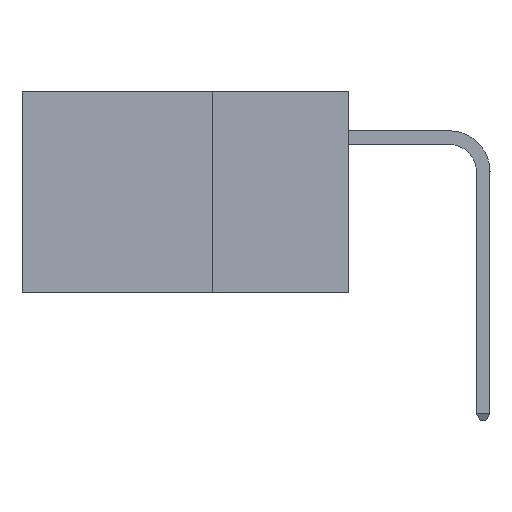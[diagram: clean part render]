
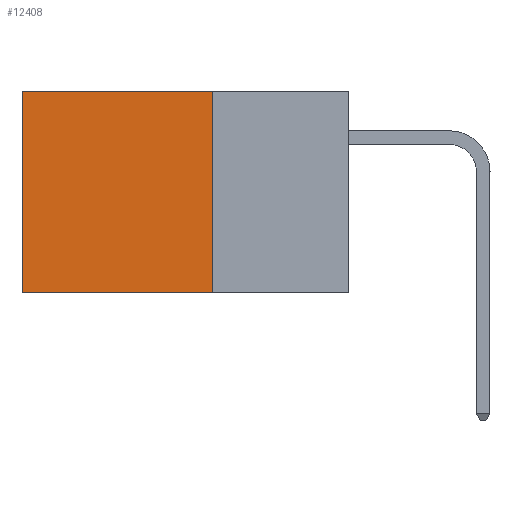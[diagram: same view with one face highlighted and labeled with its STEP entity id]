
A CAD part, left-side view. The second image highlights one B-rep face of the part: STEP entity #12408.
In plain terms, the highlighted planar face has unit normal (-1, 0, 0).
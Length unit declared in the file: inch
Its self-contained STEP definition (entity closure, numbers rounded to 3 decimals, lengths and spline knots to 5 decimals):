
#170 = ORIENTED_EDGE ( 'NONE', *, *, #18555, .F. ) ;
#573 = PLANE ( 'NONE',  #17399 ) ;
#2925 = VECTOR ( 'NONE', #14202, 39.37008 ) ;
#3123 = CARTESIAN_POINT ( 'NONE',  ( 0.2875, 0.25, 0. ) ) ;
#3824 = VECTOR ( 'NONE', #7784, 39.37008 ) ;
#4031 = EDGE_CURVE ( 'NONE', #7311, #18644, #6865, .T. ) ;
#4388 = LINE ( 'NONE', #3123, #8289 ) ;
#5728 = EDGE_CURVE ( 'NONE', #7311, #11360, #4388, .T. ) ;
#6865 = LINE ( 'NONE', #9931, #2925 ) ;
#7175 = CARTESIAN_POINT ( 'NONE',  ( 0.2875, 0.25, -0.37 ) ) ;
#7311 = VERTEX_POINT ( 'NONE', #15298 ) ;
#7784 = DIRECTION ( 'NONE',  ( 0., 1., 0. ) ) ;
#8061 = DIRECTION ( 'NONE',  ( 1., 0., 0. ) ) ;
#8214 = ORIENTED_EDGE ( 'NONE', *, *, #5728, .F. ) ;
#8289 = VECTOR ( 'NONE', #11822, 39.37008 ) ;
#9931 = CARTESIAN_POINT ( 'NONE',  ( 0.2875, 0.25, 0. ) ) ;
#10658 = LINE ( 'NONE', #16256, #3824 ) ;
#11360 = VERTEX_POINT ( 'NONE', #7175 ) ;
#11436 = CARTESIAN_POINT ( 'NONE',  ( 0.2875, 0.6, 0. ) ) ;
#11729 = FACE_OUTER_BOUND ( 'NONE', #13783, .T. ) ;
#11822 = DIRECTION ( 'NONE',  ( 0., 0., -1. ) ) ;
#12408 = ADVANCED_FACE ( 'NONE', ( #11729 ), #573, .F. ) ;
#12698 = ORIENTED_EDGE ( 'NONE', *, *, #18350, .T. ) ;
#12772 = CARTESIAN_POINT ( 'NONE',  ( 0.2875, 0.6, -0.37 ) ) ;
#13235 = VERTEX_POINT ( 'NONE', #12772 ) ;
#13783 = EDGE_LOOP ( 'NONE', ( #12698, #170, #8214, #15871 ) ) ;
#14202 = DIRECTION ( 'NONE',  ( 0., 1., 0. ) ) ;
#14650 = LINE ( 'NONE', #11436, #17878 ) ;
#15109 = CARTESIAN_POINT ( 'NONE',  ( 0.2875, 0.6, 0. ) ) ;
#15298 = CARTESIAN_POINT ( 'NONE',  ( 0.2875, 0.25, 0. ) ) ;
#15871 = ORIENTED_EDGE ( 'NONE', *, *, #4031, .T. ) ;
#16256 = CARTESIAN_POINT ( 'NONE',  ( 0.2875, 0.25, -0.37 ) ) ;
#16524 = CARTESIAN_POINT ( 'NONE',  ( 0.2875, 0.25, 0. ) ) ;
#17399 = AXIS2_PLACEMENT_3D ( 'NONE', #16524, #8061, #17902 ) ;
#17878 = VECTOR ( 'NONE', #18504, 39.37008 ) ;
#17902 = DIRECTION ( 'NONE',  ( 0., 0., -1. ) ) ;
#18350 = EDGE_CURVE ( 'NONE', #18644, #13235, #14650, .T. ) ;
#18504 = DIRECTION ( 'NONE',  ( 0., 0., -1. ) ) ;
#18555 = EDGE_CURVE ( 'NONE', #11360, #13235, #10658, .T. ) ;
#18644 = VERTEX_POINT ( 'NONE', #15109 ) ;
